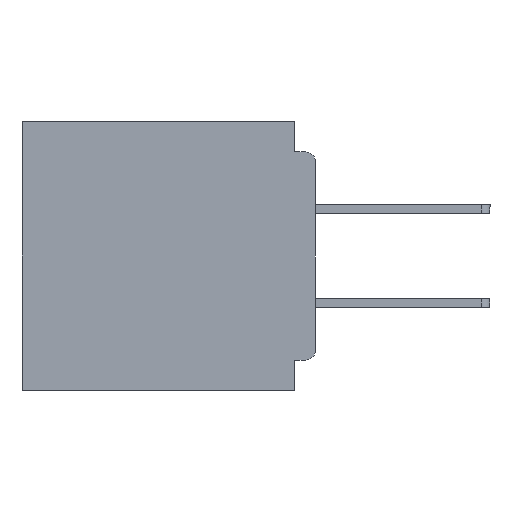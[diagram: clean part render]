
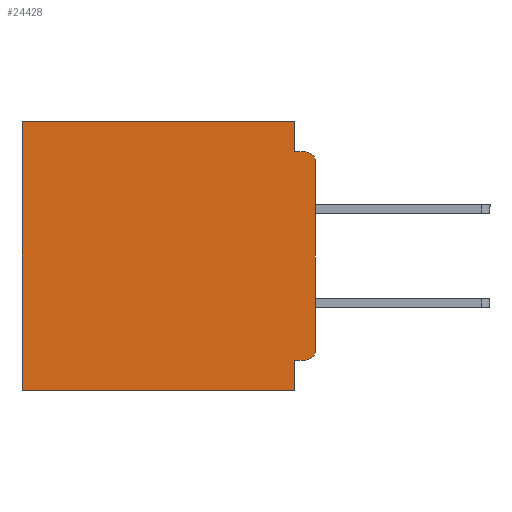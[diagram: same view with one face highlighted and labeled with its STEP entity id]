
A CAD part, left-side view. The second image highlights one B-rep face of the part: STEP entity #24428.
In plain terms, the highlighted planar face has unit normal (-1, 0, 0).
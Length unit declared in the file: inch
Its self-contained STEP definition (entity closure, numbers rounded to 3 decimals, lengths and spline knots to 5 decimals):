
#385 = DIRECTION ( 'NONE',  ( -1., 0., 0. ) ) ;
#654 = VERTEX_POINT ( 'NONE', #17709 ) ;
#782 = ORIENTED_EDGE ( 'NONE', *, *, #16819, .F. ) ;
#934 = VERTEX_POINT ( 'NONE', #42060 ) ;
#1288 = LINE ( 'NONE', #56910, #23387 ) ;
#1580 = EDGE_CURVE ( 'NONE', #37747, #654, #31223, .T. ) ;
#2904 = AXIS2_PLACEMENT_3D ( 'NONE', #26821, #385, #31226 ) ;
#3011 = EDGE_CURVE ( 'NONE', #32291, #14200, #23555, .T. ) ;
#3480 = VECTOR ( 'NONE', #5274, 39.37008 ) ;
#5274 = DIRECTION ( 'NONE',  ( 0., 1., 0. ) ) ;
#7953 = CARTESIAN_POINT ( 'NONE',  ( 0.3, 0.437, -0.4 ) ) ;
#7961 = ORIENTED_EDGE ( 'NONE', *, *, #25932, .F. ) ;
#8194 = VERTEX_POINT ( 'NONE', #7953 ) ;
#8581 = PLANE ( 'NONE',  #28677 ) ;
#8790 = ORIENTED_EDGE ( 'NONE', *, *, #3011, .F. ) ;
#9026 = LINE ( 'NONE', #31947, #18011 ) ;
#9197 = CARTESIAN_POINT ( 'NONE',  ( 0.3, 0., -0.06 ) ) ;
#10348 = CIRCLE ( 'NONE', #41759, 0.015 ) ;
#10614 = CARTESIAN_POINT ( 'NONE',  ( 0.3, 0.031, 0. ) ) ;
#12613 = CARTESIAN_POINT ( 'NONE',  ( 0.3, 0.015, -0.34 ) ) ;
#13567 = VECTOR ( 'NONE', #15058, 39.37008 ) ;
#13840 = ORIENTED_EDGE ( 'NONE', *, *, #15726, .F. ) ;
#14200 = VERTEX_POINT ( 'NONE', #26038 ) ;
#14239 = DIRECTION ( 'NONE',  ( 0., 1., 0. ) ) ;
#14368 = VECTOR ( 'NONE', #24028, 39.37008 ) ;
#14440 = LINE ( 'NONE', #44279, #36494 ) ;
#14823 = CARTESIAN_POINT ( 'NONE',  ( 0.3, 0., -0.4 ) ) ;
#15058 = DIRECTION ( 'NONE',  ( 0., 0., -1. ) ) ;
#15726 = EDGE_CURVE ( 'NONE', #27694, #8194, #25584, .T. ) ;
#15733 = ORIENTED_EDGE ( 'NONE', *, *, #38743, .T. ) ;
#16478 = CIRCLE ( 'NONE', #2904, 0.015 ) ;
#16819 = EDGE_CURVE ( 'NONE', #934, #27694, #14440, .T. ) ;
#16965 = ORIENTED_EDGE ( 'NONE', *, *, #50915, .T. ) ;
#17027 = DIRECTION ( 'NONE',  ( 0., 0., -1. ) ) ;
#17487 = CARTESIAN_POINT ( 'NONE',  ( 0.3, 0., -0.4 ) ) ;
#17709 = CARTESIAN_POINT ( 'NONE',  ( 0.3, 0., -0.34 ) ) ;
#17952 = DIRECTION ( 'NONE',  ( 0., 0., -1. ) ) ;
#18011 = VECTOR ( 'NONE', #14239, 39.37008 ) ;
#18141 = VECTOR ( 'NONE', #34486, 39.37008 ) ;
#19781 = EDGE_CURVE ( 'NONE', #25289, #32291, #25252, .T. ) ;
#21781 = CARTESIAN_POINT ( 'NONE',  ( 0.3, 0.015, -0.355 ) ) ;
#22299 = CARTESIAN_POINT ( 'NONE',  ( 0.3, 0.437, 0. ) ) ;
#23387 = VECTOR ( 'NONE', #48314, 39.37008 ) ;
#23555 = LINE ( 'NONE', #37001, #45572 ) ;
#24028 = DIRECTION ( 'NONE',  ( 0., 0., -1. ) ) ;
#24428 = ADVANCED_FACE ( 'NONE', ( #53558 ), #8581, .F. ) ;
#25252 = LINE ( 'NONE', #10614, #13567 ) ;
#25289 = VERTEX_POINT ( 'NONE', #32012 ) ;
#25584 = LINE ( 'NONE', #53609, #3480 ) ;
#25932 = EDGE_CURVE ( 'NONE', #49493, #934, #9026, .T. ) ;
#26038 = CARTESIAN_POINT ( 'NONE',  ( 0.3, 0.015, -0.045 ) ) ;
#26336 = DIRECTION ( 'NONE',  ( 1., 0., 0. ) ) ;
#26413 = CARTESIAN_POINT ( 'NONE',  ( 0.3, 0.031, -0.045 ) ) ;
#26821 = CARTESIAN_POINT ( 'NONE',  ( 0.3, 0.015, -0.06 ) ) ;
#27366 = EDGE_CURVE ( 'NONE', #37747, #14200, #16478, .T. ) ;
#27460 = EDGE_LOOP ( 'NONE', ( #45096, #44455, #8790, #36274, #16965, #39026, #13840, #782, #7961, #15733 ) ) ;
#27694 = VERTEX_POINT ( 'NONE', #37965 ) ;
#28219 = EDGE_CURVE ( 'NONE', #53643, #8194, #49489, .T. ) ;
#28424 = CARTESIAN_POINT ( 'NONE',  ( 0.3, 0.437, -0.4 ) ) ;
#28677 = AXIS2_PLACEMENT_3D ( 'NONE', #17487, #26336, #43023 ) ;
#31223 = LINE ( 'NONE', #14823, #18141 ) ;
#31226 = DIRECTION ( 'NONE',  ( 0., 0., -1. ) ) ;
#31947 = CARTESIAN_POINT ( 'NONE',  ( 0.3, 0., -0.355 ) ) ;
#32012 = CARTESIAN_POINT ( 'NONE',  ( 0.3, 0.031, 0. ) ) ;
#32291 = VERTEX_POINT ( 'NONE', #26413 ) ;
#34486 = DIRECTION ( 'NONE',  ( 0., 0., -1. ) ) ;
#36274 = ORIENTED_EDGE ( 'NONE', *, *, #19781, .F. ) ;
#36494 = VECTOR ( 'NONE', #17952, 39.37008 ) ;
#37001 = CARTESIAN_POINT ( 'NONE',  ( 0.3, 0., -0.045 ) ) ;
#37747 = VERTEX_POINT ( 'NONE', #9197 ) ;
#37965 = CARTESIAN_POINT ( 'NONE',  ( 0.3, 0.031, -0.4 ) ) ;
#38743 = EDGE_CURVE ( 'NONE', #49493, #654, #10348, .T. ) ;
#39026 = ORIENTED_EDGE ( 'NONE', *, *, #28219, .T. ) ;
#41759 = AXIS2_PLACEMENT_3D ( 'NONE', #12613, #43392, #17027 ) ;
#42060 = CARTESIAN_POINT ( 'NONE',  ( 0.3, 0.031, -0.355 ) ) ;
#43023 = DIRECTION ( 'NONE',  ( 0., 0., -1. ) ) ;
#43392 = DIRECTION ( 'NONE',  ( -1., 0., 0. ) ) ;
#44279 = CARTESIAN_POINT ( 'NONE',  ( 0.3, 0.031, -0.4 ) ) ;
#44455 = ORIENTED_EDGE ( 'NONE', *, *, #27366, .T. ) ;
#45096 = ORIENTED_EDGE ( 'NONE', *, *, #1580, .F. ) ;
#45145 = DIRECTION ( 'NONE',  ( 0., -1., 0. ) ) ;
#45572 = VECTOR ( 'NONE', #45145, 39.37008 ) ;
#48314 = DIRECTION ( 'NONE',  ( 0., 1., 0. ) ) ;
#49489 = LINE ( 'NONE', #28424, #14368 ) ;
#49493 = VERTEX_POINT ( 'NONE', #21781 ) ;
#50915 = EDGE_CURVE ( 'NONE', #25289, #53643, #1288, .T. ) ;
#53558 = FACE_OUTER_BOUND ( 'NONE', #27460, .T. ) ;
#53609 = CARTESIAN_POINT ( 'NONE',  ( 0.3, 0., -0.4 ) ) ;
#53643 = VERTEX_POINT ( 'NONE', #22299 ) ;
#56910 = CARTESIAN_POINT ( 'NONE',  ( 0.3, 0., 0. ) ) ;
